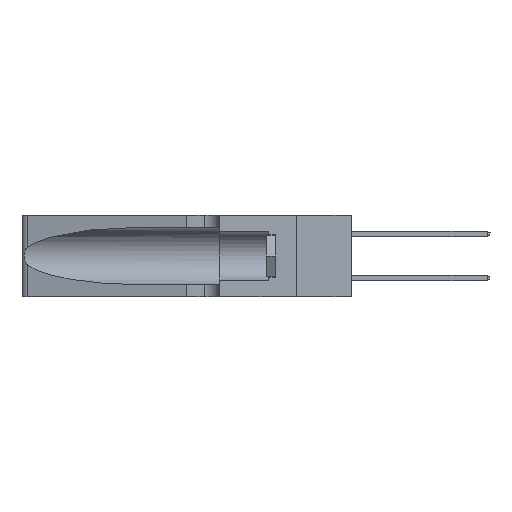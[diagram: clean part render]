
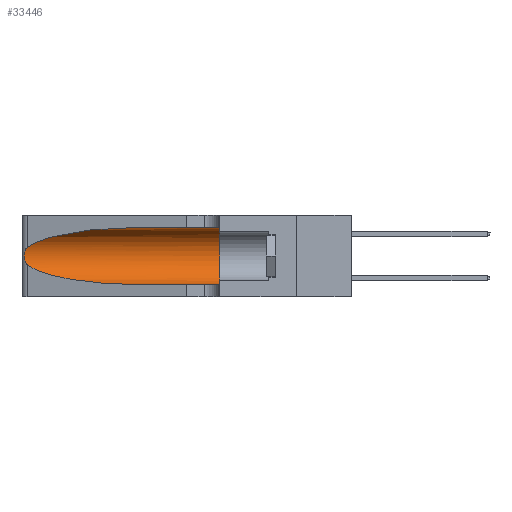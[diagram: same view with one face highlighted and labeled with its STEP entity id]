
A CAD part, left-side view. The second image highlights one B-rep face of the part: STEP entity #33446.
In plain terms, the highlighted cylindrical face has radius 3.308 mm (diameter 6.617 mm), a partial arc.
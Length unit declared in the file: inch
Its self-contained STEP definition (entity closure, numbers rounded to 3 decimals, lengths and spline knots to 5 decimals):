
#329 = CARTESIAN_POINT ( 'NONE',  ( 0.25639, 1.23184, 0.21858 ) ) ;
#1215 = EDGE_CURVE ( 'NONE', #19411, #26810, #26012, .T. ) ;
#1426 = CYLINDRICAL_SURFACE ( 'NONE', #2657, 0.13025 ) ;
#1644 = CARTESIAN_POINT ( 'NONE',  ( 0.25487, 1.22718, 0.22369 ) ) ;
#2657 = AXIS2_PLACEMENT_3D ( 'NONE', #27524, #29983, #6656 ) ;
#3027 = CARTESIAN_POINT ( 'NONE',  ( 0.25854, 1.2359, 0.20912 ) ) ;
#3034 = CARTESIAN_POINT ( 'NONE',  ( 0.18966, 0.96281, 0.05475 ) ) ;
#3347 = VECTOR ( 'NONE', #33158, 39.37008 ) ;
#4706 = CARTESIAN_POINT ( 'NONE',  ( 0.1305, 0.35, 0.31525 ) ) ;
#4877 = VERTEX_POINT ( 'NONE', #1644 ) ;
#4948 = VERTEX_POINT ( 'NONE', #4706 ) ;
#5280 = DIRECTION ( 'NONE',  ( 0., 1., 0. ) ) ;
#5550 = EDGE_CURVE ( 'NONE', #26477, #4877, #17400, .T. ) ;
#5706 = CARTESIAN_POINT ( 'NONE',  ( 0.26075, 1.23896, 0.19203 ) ) ;
#6656 = DIRECTION ( 'NONE',  ( 0., 0., -1. ) ) ;
#7105 = CARTESIAN_POINT ( 'NONE',  ( 0.1305, 1.61858, 0.31525 ) ) ;
#8099 = ORIENTED_EDGE ( 'NONE', *, *, #18668, .T. ) ;
#8344 = CARTESIAN_POINT ( 'NONE',  ( 0.26017, 1.23833, 0.17102 ) ) ;
#9154 = DIRECTION ( 'NONE',  ( 0., -1., 0. ) ) ;
#9313 = FACE_OUTER_BOUND ( 'NONE', #15465, .T. ) ;
#10049 = EDGE_CURVE ( 'NONE', #4877, #19315, #10488, .T. ) ;
#10458 = CARTESIAN_POINT ( 'NONE',  ( 0.1305, 0.72297, 0.31525 ) ) ;
#10488 = B_SPLINE_CURVE_WITH_KNOTS ( 'NONE', 3,
 ( #31678, #21224, #329, #18718, #3027, #21337, #5706, #23984, #8344, #26600, #10984, #29165, #13575, #31784 ),
 .UNSPECIFIED., .F., .F.,
 ( 4, 2, 2, 2, 2, 2, 4 ),
 ( 0., 0.00027, 0.00053, 0.00107, 0.0016, 0.00187, 0.00214 ),
 .UNSPECIFIED. ) ;
#10797 = AXIS2_PLACEMENT_3D ( 'NONE', #20924, #5280, #23565 ) ;
#10984 = CARTESIAN_POINT ( 'NONE',  ( 0.25789, 1.23486, 0.15765 ) ) ;
#11754 = CARTESIAN_POINT ( 'NONE',  ( 0.1305, 0.72297, 0.05475 ) ) ;
#12608 = ORIENTED_EDGE ( 'NONE', *, *, #5550, .T. ) ;
#12672 = CARTESIAN_POINT ( 'NONE',  ( 0.1305, 0.72297, 0.31525 ) ) ;
#13575 = CARTESIAN_POINT ( 'NONE',  ( 0.25555, 1.22993, 0.14849 ) ) ;
#14345 = CIRCLE ( 'NONE', #10797, 0.13025 ) ;
#15297 = CARTESIAN_POINT ( 'NONE',  ( 0.18966, 0.96281, 0.31525 ) ) ;
#15465 = EDGE_LOOP ( 'NONE', ( #12608, #17458, #8099, #16497, #31230, #18534 ) ) ;
#16113 = CARTESIAN_POINT ( 'NONE',  ( 0.2373, 1.15595, 0.08982 ) ) ;
#16484 = EDGE_CURVE ( 'NONE', #26477, #4948, #18930, .T. ) ;
#16497 = ORIENTED_EDGE ( 'NONE', *, *, #1215, .T. ) ;
#16915 = CARTESIAN_POINT ( 'NONE',  ( 0.1305, 1.61858, 0.05475 ) ) ;
#17400 =( BOUNDED_CURVE ( )  B_SPLINE_CURVE ( 3, ( #12672, #15297, #33467, #17943 ),
 .UNSPECIFIED., .F., .T. ) 
 B_SPLINE_CURVE_WITH_KNOTS ( ( 4, 4 ),
 ( 1.5708, 2.84003 ),
 .UNSPECIFIED. ) 
 CURVE ( )  GEOMETRIC_REPRESENTATION_ITEM ( )  RATIONAL_B_SPLINE_CURVE ( ( 1., 0.87, 0.87, 1. ) ) 
 REPRESENTATION_ITEM ( '' )  );
#17458 = ORIENTED_EDGE ( 'NONE', *, *, #10049, .T. ) ;
#17943 = CARTESIAN_POINT ( 'NONE',  ( 0.25487, 1.22718, 0.22369 ) ) ;
#18534 = ORIENTED_EDGE ( 'NONE', *, *, #16484, .F. ) ;
#18668 = EDGE_CURVE ( 'NONE', #19315, #19411, #26170, .T. ) ;
#18718 = CARTESIAN_POINT ( 'NONE',  ( 0.25787, 1.23484, 0.2124 ) ) ;
#18930 = LINE ( 'NONE', #7105, #3347 ) ;
#19315 = VERTEX_POINT ( 'NONE', #29484 ) ;
#19411 = VERTEX_POINT ( 'NONE', #11754 ) ;
#20924 = CARTESIAN_POINT ( 'NONE',  ( 0.1305, 0.35, 0.185 ) ) ;
#21224 = CARTESIAN_POINT ( 'NONE',  ( 0.25555, 1.22994, 0.2215 ) ) ;
#21232 = CARTESIAN_POINT ( 'NONE',  ( 0.25487, 1.22718, 0.14631 ) ) ;
#21337 = CARTESIAN_POINT ( 'NONE',  ( 0.26018, 1.23835, 0.19895 ) ) ;
#21350 = CARTESIAN_POINT ( 'NONE',  ( 0.1305, 0.72297, 0.05475 ) ) ;
#23565 = DIRECTION ( 'NONE',  ( 0., 0., 1. ) ) ;
#23984 = CARTESIAN_POINT ( 'NONE',  ( 0.26075, 1.23896, 0.178 ) ) ;
#24920 = CARTESIAN_POINT ( 'NONE',  ( 0.1305, 0.35, 0.05475 ) ) ;
#26012 = LINE ( 'NONE', #16915, #32861 ) ;
#26170 =( BOUNDED_CURVE ( )  B_SPLINE_CURVE ( 3, ( #21232, #16113, #3034, #21350 ),
 .UNSPECIFIED., .F., .F. ) 
 B_SPLINE_CURVE_WITH_KNOTS ( ( 4, 4 ),
 ( 3.44316, 4.71239 ),
 .UNSPECIFIED. ) 
 CURVE ( )  GEOMETRIC_REPRESENTATION_ITEM ( )  RATIONAL_B_SPLINE_CURVE ( ( 1., 0.87, 0.87, 1. ) ) 
 REPRESENTATION_ITEM ( '' )  );
#26477 = VERTEX_POINT ( 'NONE', #10458 ) ;
#26600 = CARTESIAN_POINT ( 'NONE',  ( 0.25856, 1.23593, 0.16098 ) ) ;
#26810 = VERTEX_POINT ( 'NONE', #24920 ) ;
#27524 = CARTESIAN_POINT ( 'NONE',  ( 0.1305, 1.61858, 0.185 ) ) ;
#29165 = CARTESIAN_POINT ( 'NONE',  ( 0.25639, 1.23186, 0.15144 ) ) ;
#29484 = CARTESIAN_POINT ( 'NONE',  ( 0.25487, 1.22718, 0.14631 ) ) ;
#29983 = DIRECTION ( 'NONE',  ( 0., -1., 0. ) ) ;
#31105 = EDGE_CURVE ( 'NONE', #4948, #26810, #14345, .T. ) ;
#31230 = ORIENTED_EDGE ( 'NONE', *, *, #31105, .F. ) ;
#31678 = CARTESIAN_POINT ( 'NONE',  ( 0.25487, 1.22718, 0.22369 ) ) ;
#31784 = CARTESIAN_POINT ( 'NONE',  ( 0.25487, 1.22718, 0.14631 ) ) ;
#32861 = VECTOR ( 'NONE', #9154, 39.37008 ) ;
#33158 = DIRECTION ( 'NONE',  ( 0., -1., 0. ) ) ;
#33446 = ADVANCED_FACE ( 'NONE', ( #9313 ), #1426, .F. ) ;
#33467 = CARTESIAN_POINT ( 'NONE',  ( 0.2373, 1.15595, 0.28018 ) ) ;
